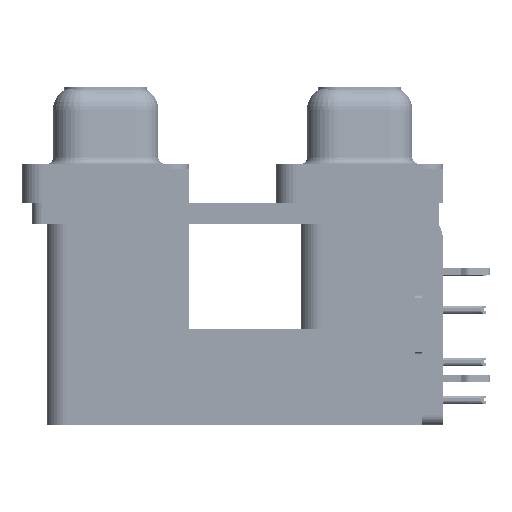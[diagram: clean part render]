
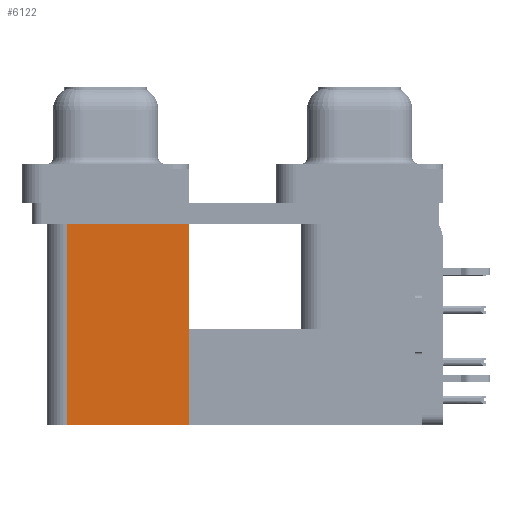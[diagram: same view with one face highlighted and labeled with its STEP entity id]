
A CAD part, left-side view. The second image highlights one B-rep face of the part: STEP entity #6122.
In plain terms, the highlighted planar face has unit normal (-1, 0, 0).
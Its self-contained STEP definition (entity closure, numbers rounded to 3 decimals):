
#931 = EDGE_CURVE ( 'NONE', #30457, #41887, #3810, .T. ) ;
#3810 = LINE ( 'NONE', #50664, #29083 ) ;
#5628 = FACE_OUTER_BOUND ( 'NONE', #59121, .T. ) ;
#6122 = ADVANCED_FACE ( 'NONE', ( #5628 ), #16585, .F. ) ;
#8382 = CARTESIAN_POINT ( 'NONE',  ( 3.79, 21.975, -19.2 ) ) ;
#9933 = VECTOR ( 'NONE', #37888, 1000. ) ;
#11876 = DIRECTION ( 'NONE',  ( 0., 0., -1. ) ) ;
#13992 = CARTESIAN_POINT ( 'NONE',  ( 3.79, 21.975, -2.5 ) ) ;
#14693 = ORIENTED_EDGE ( 'NONE', *, *, #931, .F. ) ;
#16585 = PLANE ( 'NONE',  #21393 ) ;
#17093 = LINE ( 'NONE', #58097, #36466 ) ;
#19345 = LINE ( 'NONE', #49411, #58098 ) ;
#21393 = AXIS2_PLACEMENT_3D ( 'NONE', #70788, #41919, #11876 ) ;
#26180 = LINE ( 'NONE', #67124, #9933 ) ;
#26622 = EDGE_CURVE ( 'NONE', #38610, #50193, #17093, .T. ) ;
#27756 = ORIENTED_EDGE ( 'NONE', *, *, #62849, .F. ) ;
#29083 = VECTOR ( 'NONE', #51427, 1000. ) ;
#30457 = VERTEX_POINT ( 'NONE', #8382 ) ;
#32426 = EDGE_CURVE ( 'NONE', #50193, #41887, #19345, .T. ) ;
#35590 = CARTESIAN_POINT ( 'NONE',  ( 3.79, 12.775, -2.5 ) ) ;
#36466 = VECTOR ( 'NONE', #51470, 1000. ) ;
#37888 = DIRECTION ( 'NONE',  ( 0., 1., 0. ) ) ;
#38610 = VERTEX_POINT ( 'NONE', #73343 ) ;
#39667 = ORIENTED_EDGE ( 'NONE', *, *, #32426, .T. ) ;
#41887 = VERTEX_POINT ( 'NONE', #13992 ) ;
#41919 = DIRECTION ( 'NONE',  ( 1., 0., 0. ) ) ;
#49411 = CARTESIAN_POINT ( 'NONE',  ( 3.79, 12.775, -2.5 ) ) ;
#50193 = VERTEX_POINT ( 'NONE', #35590 ) ;
#50664 = CARTESIAN_POINT ( 'NONE',  ( 3.79, 21.975, -19.2 ) ) ;
#51427 = DIRECTION ( 'NONE',  ( 0., 0., 1. ) ) ;
#51470 = DIRECTION ( 'NONE',  ( 0., 0., 1. ) ) ;
#55916 = ORIENTED_EDGE ( 'NONE', *, *, #26622, .T. ) ;
#58097 = CARTESIAN_POINT ( 'NONE',  ( 3.79, 12.775, -19.2 ) ) ;
#58098 = VECTOR ( 'NONE', #67713, 1000. ) ;
#59121 = EDGE_LOOP ( 'NONE', ( #39667, #14693, #27756, #55916 ) ) ;
#62849 = EDGE_CURVE ( 'NONE', #38610, #30457, #26180, .T. ) ;
#67124 = CARTESIAN_POINT ( 'NONE',  ( 3.79, 12.775, -19.2 ) ) ;
#67713 = DIRECTION ( 'NONE',  ( 0., 1., 0. ) ) ;
#70788 = CARTESIAN_POINT ( 'NONE',  ( 3.79, 12.775, -19.2 ) ) ;
#73343 = CARTESIAN_POINT ( 'NONE',  ( 3.79, 12.775, -19.2 ) ) ;
